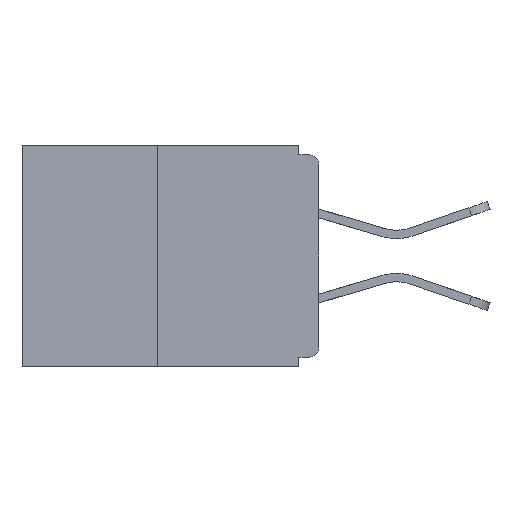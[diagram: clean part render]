
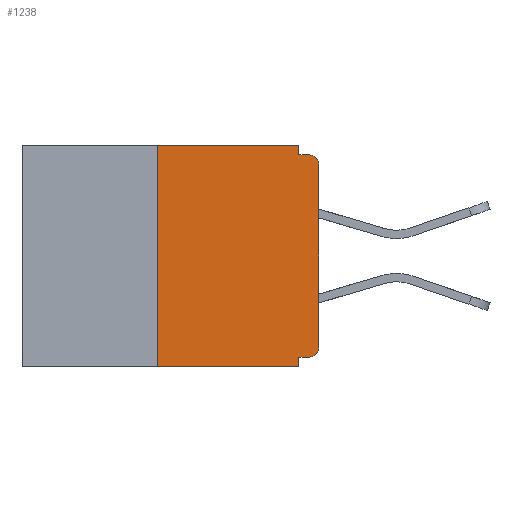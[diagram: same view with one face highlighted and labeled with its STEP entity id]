
A CAD part, left-side view. The second image highlights one B-rep face of the part: STEP entity #1238.
In plain terms, the highlighted planar face has unit normal (-1, 0, 0).
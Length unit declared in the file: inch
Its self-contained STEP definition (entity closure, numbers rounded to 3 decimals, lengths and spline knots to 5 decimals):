
#351 = EDGE_CURVE ( 'NONE', #2537, #14523, #3873, .T. ) ;
#713 = CARTESIAN_POINT ( 'NONE',  ( 0., 0.46, 0. ) ) ;
#721 = CARTESIAN_POINT ( 'NONE',  ( 0., 0., -0.313 ) ) ;
#830 = VERTEX_POINT ( 'NONE', #15626 ) ;
#1131 = CARTESIAN_POINT ( 'NONE',  ( 0., 0.031, 0. ) ) ;
#1167 = DIRECTION ( 'NONE',  ( -1., 0., 0. ) ) ;
#1238 = ADVANCED_FACE ( 'NONE', ( #12021 ), #6928, .F. ) ;
#1373 = EDGE_LOOP ( 'NONE', ( #1821, #16703, #15285, #1397, #6791, #2945, #5220, #12947, #6115, #16078 ) ) ;
#1397 = ORIENTED_EDGE ( 'NONE', *, *, #5474, .F. ) ;
#1734 = DIRECTION ( 'NONE',  ( 0., 0., -1. ) ) ;
#1821 = ORIENTED_EDGE ( 'NONE', *, *, #6061, .F. ) ;
#1918 = EDGE_CURVE ( 'NONE', #10317, #830, #7477, .T. ) ;
#2031 = VERTEX_POINT ( 'NONE', #3335 ) ;
#2385 = VECTOR ( 'NONE', #4975, 39.37008 ) ;
#2537 = VERTEX_POINT ( 'NONE', #16187 ) ;
#2702 = DIRECTION ( 'NONE',  ( 0., 0., -1. ) ) ;
#2903 = VECTOR ( 'NONE', #12436, 39.37008 ) ;
#2910 = CARTESIAN_POINT ( 'NONE',  ( 0., 0.46, 0. ) ) ;
#2945 = ORIENTED_EDGE ( 'NONE', *, *, #14023, .T. ) ;
#3145 = CARTESIAN_POINT ( 'NONE',  ( 0., 0.015, -0.328 ) ) ;
#3335 = CARTESIAN_POINT ( 'NONE',  ( 0., 0., -0.03 ) ) ;
#3376 = CARTESIAN_POINT ( 'NONE',  ( 0., 0.46, -0.343 ) ) ;
#3690 = CARTESIAN_POINT ( 'NONE',  ( 0., 0.25, 0. ) ) ;
#3864 = DIRECTION ( 'NONE',  ( 0., -1., 0. ) ) ;
#3866 = DIRECTION ( 'NONE',  ( 0., 0., -1. ) ) ;
#3873 = LINE ( 'NONE', #3376, #9559 ) ;
#4384 = DIRECTION ( 'NONE',  ( 1., 0., 0. ) ) ;
#4975 = DIRECTION ( 'NONE',  ( 0., 0., -1. ) ) ;
#5220 = ORIENTED_EDGE ( 'NONE', *, *, #9157, .T. ) ;
#5422 = CARTESIAN_POINT ( 'NONE',  ( 0., 0.015, -0.03 ) ) ;
#5432 = VECTOR ( 'NONE', #3864, 39.37008 ) ;
#5474 = EDGE_CURVE ( 'NONE', #9423, #14523, #15071, .T. ) ;
#5806 = EDGE_CURVE ( 'NONE', #2031, #10319, #16098, .T. ) ;
#5821 = VECTOR ( 'NONE', #17188, 39.37008 ) ;
#6003 = DIRECTION ( 'NONE',  ( 0., -1., 0. ) ) ;
#6061 = EDGE_CURVE ( 'NONE', #12496, #10317, #11520, .T. ) ;
#6115 = ORIENTED_EDGE ( 'NONE', *, *, #10638, .F. ) ;
#6703 = CARTESIAN_POINT ( 'NONE',  ( 0., 0., 0. ) ) ;
#6706 = CARTESIAN_POINT ( 'NONE',  ( 0., 0.031, -0.343 ) ) ;
#6791 = ORIENTED_EDGE ( 'NONE', *, *, #7691, .F. ) ;
#6928 = PLANE ( 'NONE',  #11865 ) ;
#7067 = VECTOR ( 'NONE', #1734, 39.37008 ) ;
#7477 = LINE ( 'NONE', #11157, #7067 ) ;
#7691 = EDGE_CURVE ( 'NONE', #14650, #9423, #16037, .T. ) ;
#8039 = CIRCLE ( 'NONE', #12478, 0.015 ) ;
#8175 = VERTEX_POINT ( 'NONE', #721 ) ;
#8424 = CARTESIAN_POINT ( 'NONE',  ( 0., 0., -0.328 ) ) ;
#8875 = DIRECTION ( 'NONE',  ( 0., -1., 0. ) ) ;
#9157 = EDGE_CURVE ( 'NONE', #8175, #2031, #16970, .T. ) ;
#9209 = CARTESIAN_POINT ( 'NONE',  ( 0., 0.015, -0.313 ) ) ;
#9423 = VERTEX_POINT ( 'NONE', #11801 ) ;
#9477 = AXIS2_PLACEMENT_3D ( 'NONE', #5422, #14878, #2702 ) ;
#9559 = VECTOR ( 'NONE', #6003, 39.37008 ) ;
#9846 = DIRECTION ( 'NONE',  ( 0., 0., 1. ) ) ;
#10082 = CARTESIAN_POINT ( 'NONE',  ( 0., 0.25, 0. ) ) ;
#10203 = CARTESIAN_POINT ( 'NONE',  ( 0., 0.031, -0.343 ) ) ;
#10317 = VERTEX_POINT ( 'NONE', #1131 ) ;
#10319 = VERTEX_POINT ( 'NONE', #11789 ) ;
#10638 = EDGE_CURVE ( 'NONE', #830, #10319, #16284, .T. ) ;
#11157 = CARTESIAN_POINT ( 'NONE',  ( 0., 0.031, 0. ) ) ;
#11457 = EDGE_CURVE ( 'NONE', #2537, #12496, #13145, .T. ) ;
#11520 = LINE ( 'NONE', #713, #15676 ) ;
#11789 = CARTESIAN_POINT ( 'NONE',  ( 0., 0.015, -0.015 ) ) ;
#11801 = CARTESIAN_POINT ( 'NONE',  ( 0., 0.031, -0.328 ) ) ;
#11865 = AXIS2_PLACEMENT_3D ( 'NONE', #2910, #4384, #12224 ) ;
#12021 = FACE_OUTER_BOUND ( 'NONE', #1373, .T. ) ;
#12224 = DIRECTION ( 'NONE',  ( 0., 0., -1. ) ) ;
#12436 = DIRECTION ( 'NONE',  ( 0., 1., 0. ) ) ;
#12478 = AXIS2_PLACEMENT_3D ( 'NONE', #9209, #1167, #3866 ) ;
#12496 = VERTEX_POINT ( 'NONE', #10082 ) ;
#12947 = ORIENTED_EDGE ( 'NONE', *, *, #5806, .T. ) ;
#13145 = LINE ( 'NONE', #3690, #5821 ) ;
#13316 = CARTESIAN_POINT ( 'NONE',  ( 0., 0., -0.015 ) ) ;
#13846 = VECTOR ( 'NONE', #9846, 39.37008 ) ;
#14023 = EDGE_CURVE ( 'NONE', #14650, #8175, #8039, .T. ) ;
#14523 = VERTEX_POINT ( 'NONE', #6706 ) ;
#14650 = VERTEX_POINT ( 'NONE', #3145 ) ;
#14878 = DIRECTION ( 'NONE',  ( -1., 0., 0. ) ) ;
#15071 = LINE ( 'NONE', #10203, #2385 ) ;
#15285 = ORIENTED_EDGE ( 'NONE', *, *, #351, .T. ) ;
#15626 = CARTESIAN_POINT ( 'NONE',  ( 0., 0.031, -0.015 ) ) ;
#15676 = VECTOR ( 'NONE', #8875, 39.37008 ) ;
#16037 = LINE ( 'NONE', #8424, #2903 ) ;
#16078 = ORIENTED_EDGE ( 'NONE', *, *, #1918, .F. ) ;
#16098 = CIRCLE ( 'NONE', #9477, 0.015 ) ;
#16187 = CARTESIAN_POINT ( 'NONE',  ( 0., 0.25, -0.343 ) ) ;
#16284 = LINE ( 'NONE', #13316, #5432 ) ;
#16703 = ORIENTED_EDGE ( 'NONE', *, *, #11457, .F. ) ;
#16970 = LINE ( 'NONE', #6703, #13846 ) ;
#17188 = DIRECTION ( 'NONE',  ( 0., 0., 1. ) ) ;
